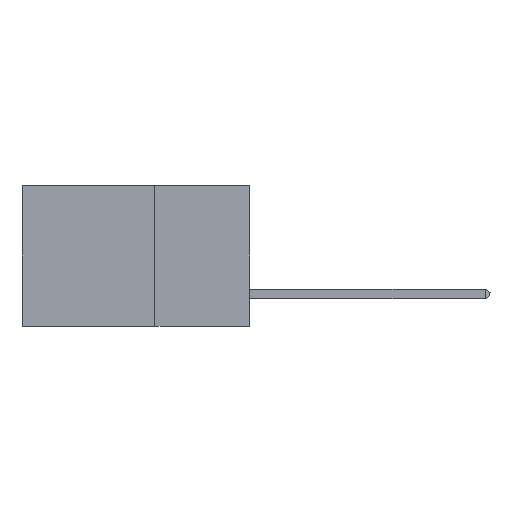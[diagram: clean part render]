
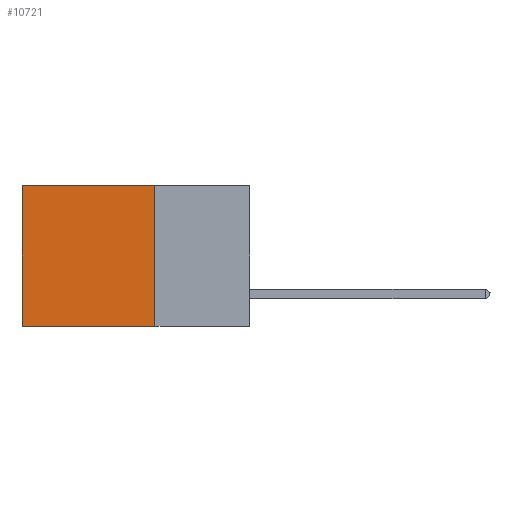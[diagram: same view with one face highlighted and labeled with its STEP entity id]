
A CAD part, left-side view. The second image highlights one B-rep face of the part: STEP entity #10721.
In plain terms, the highlighted planar face has unit normal (-1, 0, 0).
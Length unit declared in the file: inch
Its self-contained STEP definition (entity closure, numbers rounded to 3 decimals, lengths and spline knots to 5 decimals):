
#740 = DIRECTION ( 'NONE',  ( 0., 0., -1. ) ) ;
#773 = LINE ( 'NONE', #14369, #4429 ) ;
#1012 = VERTEX_POINT ( 'NONE', #11818 ) ;
#3037 = EDGE_CURVE ( 'NONE', #6782, #6000, #7481, .T. ) ;
#3245 = PLANE ( 'NONE',  #8238 ) ;
#3270 = DIRECTION ( 'NONE',  ( 0., 1., 0. ) ) ;
#3386 = DIRECTION ( 'NONE',  ( 0., 0., -1. ) ) ;
#3928 = LINE ( 'NONE', #22216, #20819 ) ;
#4134 = EDGE_LOOP ( 'NONE', ( #22662, #18183, #17822, #20538 ) ) ;
#4429 = VECTOR ( 'NONE', #24089, 39.37008 ) ;
#5226 = CARTESIAN_POINT ( 'NONE',  ( 0.2875, 0.25, 0. ) ) ;
#6000 = VERTEX_POINT ( 'NONE', #7237 ) ;
#6782 = VERTEX_POINT ( 'NONE', #20549 ) ;
#7237 = CARTESIAN_POINT ( 'NONE',  ( 0.2875, 0.6, 0. ) ) ;
#7350 = DIRECTION ( 'NONE',  ( 1., 0., 0. ) ) ;
#7385 = CARTESIAN_POINT ( 'NONE',  ( 0.2875, 0.25, 0. ) ) ;
#7481 = LINE ( 'NONE', #7385, #23879 ) ;
#7749 = DIRECTION ( 'NONE',  ( 0., 1., 0. ) ) ;
#8238 = AXIS2_PLACEMENT_3D ( 'NONE', #5226, #7350, #3386 ) ;
#9627 = CARTESIAN_POINT ( 'NONE',  ( 0.2875, 0.25, -0.37 ) ) ;
#10115 = CARTESIAN_POINT ( 'NONE',  ( 0.2875, 0.25, -0.37 ) ) ;
#10652 = LINE ( 'NONE', #9627, #12193 ) ;
#10721 = ADVANCED_FACE ( 'NONE', ( #20057 ), #3245, .F. ) ;
#11818 = CARTESIAN_POINT ( 'NONE',  ( 0.2875, 0.6, -0.37 ) ) ;
#12193 = VECTOR ( 'NONE', #7749, 39.37008 ) ;
#14369 = CARTESIAN_POINT ( 'NONE',  ( 0.2875, 0.25, 0. ) ) ;
#17822 = ORIENTED_EDGE ( 'NONE', *, *, #20570, .F. ) ;
#18183 = ORIENTED_EDGE ( 'NONE', *, *, #18227, .F. ) ;
#18227 = EDGE_CURVE ( 'NONE', #22914, #1012, #10652, .T. ) ;
#20057 = FACE_OUTER_BOUND ( 'NONE', #4134, .T. ) ;
#20538 = ORIENTED_EDGE ( 'NONE', *, *, #3037, .T. ) ;
#20549 = CARTESIAN_POINT ( 'NONE',  ( 0.2875, 0.25, 0. ) ) ;
#20570 = EDGE_CURVE ( 'NONE', #6782, #22914, #773, .T. ) ;
#20819 = VECTOR ( 'NONE', #740, 39.37008 ) ;
#22216 = CARTESIAN_POINT ( 'NONE',  ( 0.2875, 0.6, 0. ) ) ;
#22662 = ORIENTED_EDGE ( 'NONE', *, *, #24882, .T. ) ;
#22914 = VERTEX_POINT ( 'NONE', #10115 ) ;
#23879 = VECTOR ( 'NONE', #3270, 39.37008 ) ;
#24089 = DIRECTION ( 'NONE',  ( 0., 0., -1. ) ) ;
#24882 = EDGE_CURVE ( 'NONE', #6000, #1012, #3928, .T. ) ;
